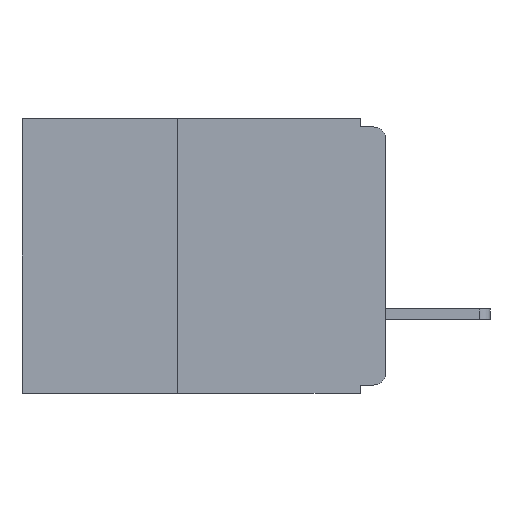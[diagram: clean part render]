
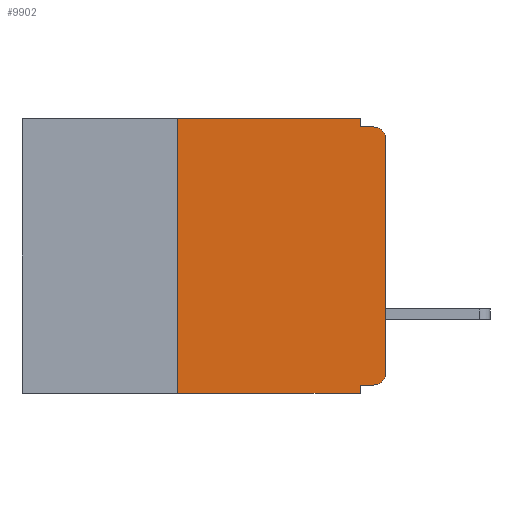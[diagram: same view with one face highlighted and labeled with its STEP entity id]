
A CAD part, left-side view. The second image highlights one B-rep face of the part: STEP entity #9902.
In plain terms, the highlighted planar face has unit normal (-1, 0, 0).
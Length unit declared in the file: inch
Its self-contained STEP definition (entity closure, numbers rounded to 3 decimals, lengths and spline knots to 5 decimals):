
#141 = AXIS2_PLACEMENT_3D ( 'NONE', #11546, #11523, #11393 ) ;
#633 = AXIS2_PLACEMENT_3D ( 'NONE', #15448, #15431, #15373 ) ;
#712 = EDGE_CURVE ( 'NONE', #2447, #16161, #860, .T. ) ;
#805 = VECTOR ( 'NONE', #2192, 39.37008 ) ;
#860 = LINE ( 'NONE', #3380, #805 ) ;
#1757 = DIRECTION ( 'NONE',  ( 0., 0., 1. ) ) ;
#2118 = CARTESIAN_POINT ( 'NONE',  ( 0., 0.25, -0.33 ) ) ;
#2192 = DIRECTION ( 'NONE',  ( 0., 0., -1. ) ) ;
#2250 = CARTESIAN_POINT ( 'NONE',  ( 0., 0., -0.01 ) ) ;
#2447 = VERTEX_POINT ( 'NONE', #16928 ) ;
#2847 = VERTEX_POINT ( 'NONE', #14080 ) ;
#2856 = VERTEX_POINT ( 'NONE', #9651 ) ;
#2944 = VERTEX_POINT ( 'NONE', #16953 ) ;
#3380 = CARTESIAN_POINT ( 'NONE',  ( 0., 0.031, -0.33 ) ) ;
#3536 = VERTEX_POINT ( 'NONE', #7853 ) ;
#4212 = AXIS2_PLACEMENT_3D ( 'NONE', #13413, #13160, #13108 ) ;
#5159 = CIRCLE ( 'NONE', #141, 0.015 ) ;
#5349 = VECTOR ( 'NONE', #14946, 39.37008 ) ;
#5597 = LINE ( 'NONE', #15389, #5349 ) ;
#6739 = ORIENTED_EDGE ( 'NONE', *, *, #17427, .T. ) ;
#6870 = ORIENTED_EDGE ( 'NONE', *, *, #10299, .T. ) ;
#6887 = ORIENTED_EDGE ( 'NONE', *, *, #17837, .F. ) ;
#7066 = EDGE_LOOP ( 'NONE', ( #6739, #6870, #6887, #7073, #7214, #7253, #7368, #7420, #7665, #7669 ) ) ;
#7073 = ORIENTED_EDGE ( 'NONE', *, *, #15266, .F. ) ;
#7214 = ORIENTED_EDGE ( 'NONE', *, *, #14575, .F. ) ;
#7253 = ORIENTED_EDGE ( 'NONE', *, *, #17841, .F. ) ;
#7368 = ORIENTED_EDGE ( 'NONE', *, *, #18116, .T. ) ;
#7420 = ORIENTED_EDGE ( 'NONE', *, *, #712, .F. ) ;
#7665 = ORIENTED_EDGE ( 'NONE', *, *, #9823, .F. ) ;
#7669 = ORIENTED_EDGE ( 'NONE', *, *, #11977, .T. ) ;
#7750 = CARTESIAN_POINT ( 'NONE',  ( 0., 0.031, 0. ) ) ;
#7853 = CARTESIAN_POINT ( 'NONE',  ( 0., 0.031, -0.01 ) ) ;
#8013 = VERTEX_POINT ( 'NONE', #15010 ) ;
#8022 = CARTESIAN_POINT ( 'NONE',  ( 0., 0.25, 0. ) ) ;
#8034 = VECTOR ( 'NONE', #17219, 39.37008 ) ;
#8071 = LINE ( 'NONE', #16569, #8034 ) ;
#9651 = CARTESIAN_POINT ( 'NONE',  ( 0., 0., -0.025 ) ) ;
#9823 = EDGE_CURVE ( 'NONE', #8013, #2447, #13484, .T. ) ;
#9856 = VECTOR ( 'NONE', #17218, 39.37008 ) ;
#9902 = ADVANCED_FACE ( 'NONE', ( #12960 ), #13731, .F. ) ;
#9960 = LINE ( 'NONE', #16319, #9856 ) ;
#10299 = EDGE_CURVE ( 'NONE', #2856, #13443, #11630, .T. ) ;
#10381 = DIRECTION ( 'NONE',  ( 0., 0., 1. ) ) ;
#10388 = CARTESIAN_POINT ( 'NONE',  ( 0., 0., 0. ) ) ;
#11175 = VECTOR ( 'NONE', #1757, 39.37008 ) ;
#11273 = CARTESIAN_POINT ( 'NONE',  ( 0., 0.031, -0.33 ) ) ;
#11327 = VECTOR ( 'NONE', #15780, 39.37008 ) ;
#11393 = DIRECTION ( 'NONE',  ( 0., 0., -1. ) ) ;
#11417 = LINE ( 'NONE', #2250, #11327 ) ;
#11439 = LINE ( 'NONE', #2118, #11175 ) ;
#11523 = DIRECTION ( 'NONE',  ( -1., 0., 0. ) ) ;
#11546 = CARTESIAN_POINT ( 'NONE',  ( 0., 0.015, -0.305 ) ) ;
#11630 = CIRCLE ( 'NONE', #633, 0.015 ) ;
#11822 = CARTESIAN_POINT ( 'NONE',  ( 0., 0.015, -0.01 ) ) ;
#11977 = EDGE_CURVE ( 'NONE', #8013, #2847, #5159, .T. ) ;
#12960 = FACE_OUTER_BOUND ( 'NONE', #7066, .T. ) ;
#13103 = VECTOR ( 'NONE', #10381, 39.37008 ) ;
#13108 = DIRECTION ( 'NONE',  ( 0., 0., -1. ) ) ;
#13160 = DIRECTION ( 'NONE',  ( 1., 0., 0. ) ) ;
#13336 = LINE ( 'NONE', #10388, #13103 ) ;
#13413 = CARTESIAN_POINT ( 'NONE',  ( 0., 0.437, 0. ) ) ;
#13443 = VERTEX_POINT ( 'NONE', #11822 ) ;
#13484 = LINE ( 'NONE', #18227, #13538 ) ;
#13538 = VECTOR ( 'NONE', #17407, 39.37008 ) ;
#13731 = PLANE ( 'NONE',  #4212 ) ;
#14080 = CARTESIAN_POINT ( 'NONE',  ( 0., 0., -0.305 ) ) ;
#14575 = EDGE_CURVE ( 'NONE', #16397, #17572, #8071, .T. ) ;
#14946 = DIRECTION ( 'NONE',  ( 0., 0., -1. ) ) ;
#15010 = CARTESIAN_POINT ( 'NONE',  ( 0., 0.015, -0.32 ) ) ;
#15266 = EDGE_CURVE ( 'NONE', #17572, #3536, #5597, .T. ) ;
#15373 = DIRECTION ( 'NONE',  ( 0., 0., -1. ) ) ;
#15389 = CARTESIAN_POINT ( 'NONE',  ( 0., 0.031, 0. ) ) ;
#15431 = DIRECTION ( 'NONE',  ( -1., 0., 0. ) ) ;
#15448 = CARTESIAN_POINT ( 'NONE',  ( 0., 0.015, -0.025 ) ) ;
#15780 = DIRECTION ( 'NONE',  ( 0., -1., 0. ) ) ;
#16161 = VERTEX_POINT ( 'NONE', #11273 ) ;
#16319 = CARTESIAN_POINT ( 'NONE',  ( 0., 0.437, -0.33 ) ) ;
#16397 = VERTEX_POINT ( 'NONE', #8022 ) ;
#16569 = CARTESIAN_POINT ( 'NONE',  ( 0., 0.437, 0. ) ) ;
#16928 = CARTESIAN_POINT ( 'NONE',  ( 0., 0.031, -0.32 ) ) ;
#16953 = CARTESIAN_POINT ( 'NONE',  ( 0., 0.25, -0.33 ) ) ;
#17218 = DIRECTION ( 'NONE',  ( 0., -1., 0. ) ) ;
#17219 = DIRECTION ( 'NONE',  ( 0., -1., 0. ) ) ;
#17407 = DIRECTION ( 'NONE',  ( 0., 1., 0. ) ) ;
#17427 = EDGE_CURVE ( 'NONE', #2847, #2856, #13336, .T. ) ;
#17572 = VERTEX_POINT ( 'NONE', #7750 ) ;
#17837 = EDGE_CURVE ( 'NONE', #3536, #13443, #11417, .T. ) ;
#17841 = EDGE_CURVE ( 'NONE', #2944, #16397, #11439, .T. ) ;
#18116 = EDGE_CURVE ( 'NONE', #2944, #16161, #9960, .T. ) ;
#18227 = CARTESIAN_POINT ( 'NONE',  ( 0., 0., -0.32 ) ) ;
